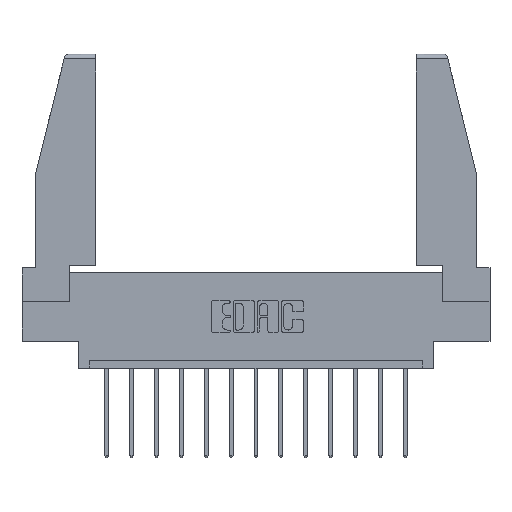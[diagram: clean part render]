
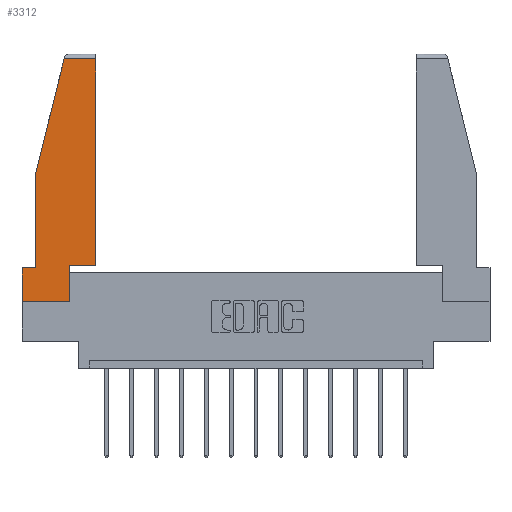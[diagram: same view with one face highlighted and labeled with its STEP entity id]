
A CAD part, top view. The second image highlights one B-rep face of the part: STEP entity #3312.
In plain terms, the highlighted planar face has unit normal (0, 0, 1).
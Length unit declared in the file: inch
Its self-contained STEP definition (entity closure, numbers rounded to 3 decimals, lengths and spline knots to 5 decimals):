
#60 = CARTESIAN_POINT ( 'NONE',  ( 0.086, 0.21, 0. ) ) ;
#713 = DIRECTION ( 'NONE',  ( 0., 0., 1. ) ) ;
#749 = ORIENTED_EDGE ( 'NONE', *, *, #6568, .T. ) ;
#802 = DIRECTION ( 'NONE',  ( 0., 1., 0. ) ) ;
#817 = DIRECTION ( 'NONE',  ( 1., 0., 0. ) ) ;
#1250 = DIRECTION ( 'NONE',  ( 1., 0., 0. ) ) ;
#1298 = ORIENTED_EDGE ( 'NONE', *, *, #5619, .T. ) ;
#1374 = FACE_OUTER_BOUND ( 'NONE', #14093, .T. ) ;
#1930 = CARTESIAN_POINT ( 'NONE',  ( 0., 0., 0. ) ) ;
#1980 = ORIENTED_EDGE ( 'NONE', *, *, #8092, .T. ) ;
#2387 = CARTESIAN_POINT ( 'NONE',  ( 0.297, 0.223, 0. ) ) ;
#2569 = LINE ( 'NONE', #15023, #4568 ) ;
#2630 = VECTOR ( 'NONE', #802, 39.37008 ) ;
#2708 = VERTEX_POINT ( 'NONE', #15449 ) ;
#3073 = VERTEX_POINT ( 'NONE', #5747 ) ;
#3274 = VECTOR ( 'NONE', #4498, 39.37008 ) ;
#3312 = ADVANCED_FACE ( 'NONE', ( #1374 ), #11350, .T. ) ;
#3381 = DIRECTION ( 'NONE',  ( 1., 0., 0. ) ) ;
#3735 = CARTESIAN_POINT ( 'NONE',  ( 0.297, 0., 0. ) ) ;
#3932 = DIRECTION ( 'NONE',  ( -0.239, -0.971, 0. ) ) ;
#4048 = CARTESIAN_POINT ( 'NONE',  ( 0., 0.21, 0. ) ) ;
#4100 = DIRECTION ( 'NONE',  ( 0., -1., 0. ) ) ;
#4498 = DIRECTION ( 'NONE',  ( -1., 0., 0. ) ) ;
#4568 = VECTOR ( 'NONE', #3932, 39.37008 ) ;
#4659 = EDGE_CURVE ( 'NONE', #15770, #13879, #7786, .T. ) ;
#4660 = CARTESIAN_POINT ( 'NONE',  ( 0.086, 0.8, 0. ) ) ;
#5083 = CARTESIAN_POINT ( 'NONE',  ( 0.461, 0.223, 0. ) ) ;
#5619 = EDGE_CURVE ( 'NONE', #9492, #10579, #7347, .T. ) ;
#5747 = CARTESIAN_POINT ( 'NONE',  ( 0.297, 0., 0. ) ) ;
#6329 = EDGE_CURVE ( 'NONE', #3073, #2708, #12123, .T. ) ;
#6564 = CARTESIAN_POINT ( 'NONE',  ( 0., 0., 0. ) ) ;
#6568 = EDGE_CURVE ( 'NONE', #12381, #15770, #9441, .T. ) ;
#7021 = ORIENTED_EDGE ( 'NONE', *, *, #9071, .T. ) ;
#7347 = LINE ( 'NONE', #4048, #10803 ) ;
#7763 = LINE ( 'NONE', #10806, #13895 ) ;
#7786 = LINE ( 'NONE', #13093, #3274 ) ;
#8092 = EDGE_CURVE ( 'NONE', #11676, #13328, #11112, .T. ) ;
#8230 = ORIENTED_EDGE ( 'NONE', *, *, #4659, .T. ) ;
#8292 = LINE ( 'NONE', #14087, #8673 ) ;
#8382 = CARTESIAN_POINT ( 'NONE',  ( 0.461, 0.223, 0. ) ) ;
#8454 = ORIENTED_EDGE ( 'NONE', *, *, #12924, .T. ) ;
#8515 = AXIS2_PLACEMENT_3D ( 'NONE', #1930, #713, #817 ) ;
#8673 = VECTOR ( 'NONE', #10464, 39.37008 ) ;
#9071 = EDGE_CURVE ( 'NONE', #13879, #11676, #2569, .T. ) ;
#9441 = LINE ( 'NONE', #8382, #2630 ) ;
#9492 = VERTEX_POINT ( 'NONE', #9716 ) ;
#9522 = LINE ( 'NONE', #2387, #14141 ) ;
#9716 = CARTESIAN_POINT ( 'NONE',  ( 0., 0.21, 0. ) ) ;
#9806 = ORIENTED_EDGE ( 'NONE', *, *, #9810, .T. ) ;
#9810 = EDGE_CURVE ( 'NONE', #13328, #9492, #8292, .T. ) ;
#10162 = ORIENTED_EDGE ( 'NONE', *, *, #6329, .T. ) ;
#10464 = DIRECTION ( 'NONE',  ( -1., 0., 0. ) ) ;
#10579 = VERTEX_POINT ( 'NONE', #6564 ) ;
#10803 = VECTOR ( 'NONE', #4100, 39.37008 ) ;
#10806 = CARTESIAN_POINT ( 'NONE',  ( 0., 0., 0. ) ) ;
#11112 = LINE ( 'NONE', #13686, #14012 ) ;
#11344 = DIRECTION ( 'NONE',  ( 0., 1., 0. ) ) ;
#11350 = PLANE ( 'NONE',  #8515 ) ;
#11676 = VERTEX_POINT ( 'NONE', #4660 ) ;
#12123 = LINE ( 'NONE', #3735, #12316 ) ;
#12316 = VECTOR ( 'NONE', #11344, 39.37008 ) ;
#12338 = ORIENTED_EDGE ( 'NONE', *, *, #14502, .T. ) ;
#12381 = VERTEX_POINT ( 'NONE', #5083 ) ;
#12605 = DIRECTION ( 'NONE',  ( 0., -1., 0. ) ) ;
#12924 = EDGE_CURVE ( 'NONE', #2708, #12381, #9522, .T. ) ;
#13093 = CARTESIAN_POINT ( 'NONE',  ( 0., 1.52, 0. ) ) ;
#13328 = VERTEX_POINT ( 'NONE', #60 ) ;
#13686 = CARTESIAN_POINT ( 'NONE',  ( 0.086, 0.8, 0. ) ) ;
#13879 = VERTEX_POINT ( 'NONE', #13925 ) ;
#13895 = VECTOR ( 'NONE', #3381, 39.37008 ) ;
#13925 = CARTESIAN_POINT ( 'NONE',  ( 0.2636, 1.52, 0. ) ) ;
#14012 = VECTOR ( 'NONE', #12605, 39.37008 ) ;
#14087 = CARTESIAN_POINT ( 'NONE',  ( 0., 0.21, 0. ) ) ;
#14093 = EDGE_LOOP ( 'NONE', ( #749, #8230, #7021, #1980, #9806, #1298, #12338, #10162, #8454 ) ) ;
#14141 = VECTOR ( 'NONE', #1250, 39.37008 ) ;
#14502 = EDGE_CURVE ( 'NONE', #10579, #3073, #7763, .T. ) ;
#15023 = CARTESIAN_POINT ( 'NONE',  ( 0.271, 1.55, 0. ) ) ;
#15130 = CARTESIAN_POINT ( 'NONE',  ( 0.461, 1.52, 0. ) ) ;
#15449 = CARTESIAN_POINT ( 'NONE',  ( 0.297, 0.223, 0. ) ) ;
#15770 = VERTEX_POINT ( 'NONE', #15130 ) ;
